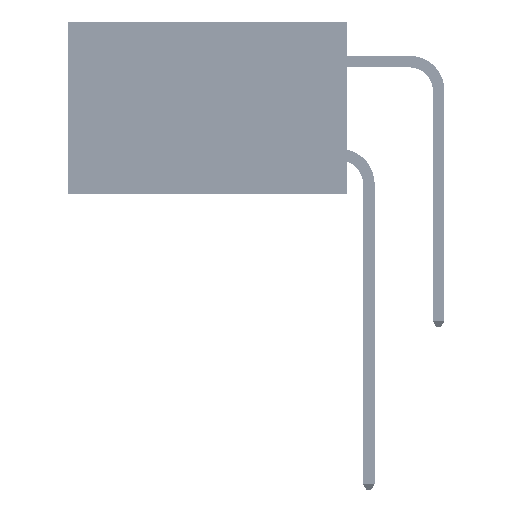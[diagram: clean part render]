
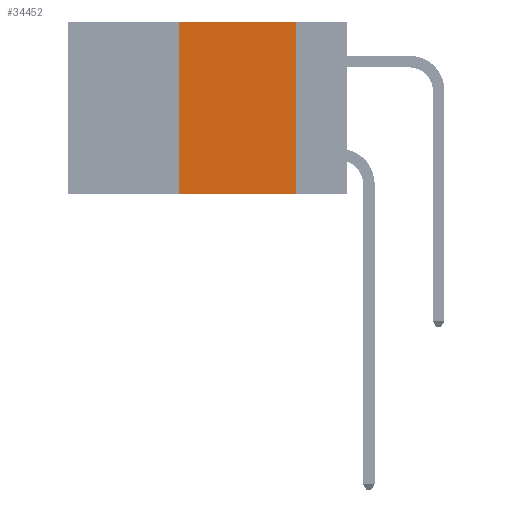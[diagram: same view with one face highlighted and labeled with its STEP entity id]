
A CAD part, left-side view. The second image highlights one B-rep face of the part: STEP entity #34452.
In plain terms, the highlighted planar face has unit normal (-1, 0, 0).
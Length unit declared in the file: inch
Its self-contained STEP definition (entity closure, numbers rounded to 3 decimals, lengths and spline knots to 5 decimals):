
#626 = AXIS2_PLACEMENT_3D ( 'NONE', #34242, #37878, #16071 ) ;
#1901 = VERTEX_POINT ( 'NONE', #27755 ) ;
#3198 = CARTESIAN_POINT ( 'NONE',  ( 0., 0.6, -0.37 ) ) ;
#3447 = CARTESIAN_POINT ( 'NONE',  ( 0., 0.36, 0. ) ) ;
#4786 = VECTOR ( 'NONE', #17729, 39.37008 ) ;
#7656 = LINE ( 'NONE', #44759, #44043 ) ;
#10419 = ORIENTED_EDGE ( 'NONE', *, *, #39676, .T. ) ;
#13669 = VECTOR ( 'NONE', #27140, 39.37008 ) ;
#13696 = LINE ( 'NONE', #3198, #30796 ) ;
#16071 = DIRECTION ( 'NONE',  ( 0., 0., -1. ) ) ;
#17665 = CARTESIAN_POINT ( 'NONE',  ( 0., 0.11, 0. ) ) ;
#17729 = DIRECTION ( 'NONE',  ( 0., 0., -1. ) ) ;
#19217 = VERTEX_POINT ( 'NONE', #20324 ) ;
#20324 = CARTESIAN_POINT ( 'NONE',  ( 0., 0.36, -0.37 ) ) ;
#21780 = ORIENTED_EDGE ( 'NONE', *, *, #29480, .F. ) ;
#24947 = CARTESIAN_POINT ( 'NONE',  ( 0., 0.11, 0. ) ) ;
#25303 = LINE ( 'NONE', #24947, #4786 ) ;
#27140 = DIRECTION ( 'NONE',  ( 0., 0., 1. ) ) ;
#27755 = CARTESIAN_POINT ( 'NONE',  ( 0., 0.11, -0.37 ) ) ;
#29210 = EDGE_CURVE ( 'NONE', #40376, #43083, #7656, .T. ) ;
#29480 = EDGE_CURVE ( 'NONE', #43083, #1901, #25303, .T. ) ;
#29843 = ORIENTED_EDGE ( 'NONE', *, *, #40702, .F. ) ;
#30796 = VECTOR ( 'NONE', #35957, 39.37008 ) ;
#31038 = EDGE_LOOP ( 'NONE', ( #21780, #45101, #29843, #10419 ) ) ;
#34018 = DIRECTION ( 'NONE',  ( 0., -1., 0. ) ) ;
#34242 = CARTESIAN_POINT ( 'NONE',  ( 0., 0.6, 0. ) ) ;
#34294 = CARTESIAN_POINT ( 'NONE',  ( 0., 0.36, 0. ) ) ;
#34452 = ADVANCED_FACE ( 'NONE', ( #40882 ), #41375, .F. ) ;
#35957 = DIRECTION ( 'NONE',  ( 0., -1., 0. ) ) ;
#37878 = DIRECTION ( 'NONE',  ( 1., 0., 0. ) ) ;
#39676 = EDGE_CURVE ( 'NONE', #19217, #1901, #13696, .T. ) ;
#40376 = VERTEX_POINT ( 'NONE', #3447 ) ;
#40702 = EDGE_CURVE ( 'NONE', #19217, #40376, #42699, .T. ) ;
#40882 = FACE_OUTER_BOUND ( 'NONE', #31038, .T. ) ;
#41375 = PLANE ( 'NONE',  #626 ) ;
#42699 = LINE ( 'NONE', #34294, #13669 ) ;
#43083 = VERTEX_POINT ( 'NONE', #17665 ) ;
#44043 = VECTOR ( 'NONE', #34018, 39.37008 ) ;
#44759 = CARTESIAN_POINT ( 'NONE',  ( 0., 0.6, 0. ) ) ;
#45101 = ORIENTED_EDGE ( 'NONE', *, *, #29210, .F. ) ;
